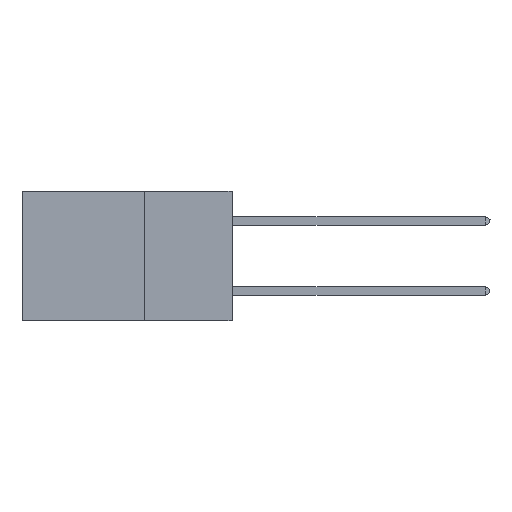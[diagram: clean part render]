
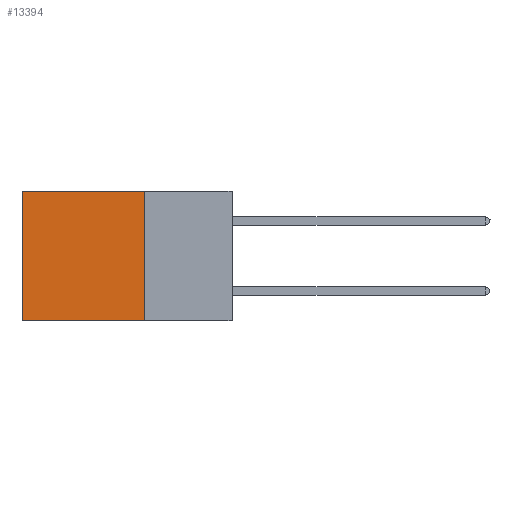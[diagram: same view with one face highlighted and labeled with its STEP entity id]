
A CAD part, left-side view. The second image highlights one B-rep face of the part: STEP entity #13394.
In plain terms, the highlighted planar face has unit normal (-1, 0, 0).
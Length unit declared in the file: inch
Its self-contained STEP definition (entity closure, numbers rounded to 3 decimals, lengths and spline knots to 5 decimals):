
#149 = CARTESIAN_POINT ( 'NONE',  ( 0.2875, 0.25, -0.37 ) ) ;
#176 = VERTEX_POINT ( 'NONE', #1480 ) ;
#900 = ORIENTED_EDGE ( 'NONE', *, *, #16935, .T. ) ;
#1480 = CARTESIAN_POINT ( 'NONE',  ( 0.2875, 0.6, -0.37 ) ) ;
#4264 = EDGE_CURVE ( 'NONE', #11045, #176, #23372, .T. ) ;
#4850 = EDGE_CURVE ( 'NONE', #27379, #11045, #20288, .T. ) ;
#5281 = CARTESIAN_POINT ( 'NONE',  ( 0.2875, 0.6, 0. ) ) ;
#5306 = VERTEX_POINT ( 'NONE', #5281 ) ;
#5441 = VECTOR ( 'NONE', #6538, 39.37008 ) ;
#5892 = ORIENTED_EDGE ( 'NONE', *, *, #22264, .T. ) ;
#6002 = CARTESIAN_POINT ( 'NONE',  ( 0.2875, 0.25, -0.37 ) ) ;
#6138 = LINE ( 'NONE', #17353, #5441 ) ;
#6538 = DIRECTION ( 'NONE',  ( 0., 0., -1. ) ) ;
#7806 = DIRECTION ( 'NONE',  ( 0., 0., -1. ) ) ;
#10648 = VECTOR ( 'NONE', #22127, 39.37008 ) ;
#11045 = VERTEX_POINT ( 'NONE', #149 ) ;
#11805 = CARTESIAN_POINT ( 'NONE',  ( 0.2875, 0.25, 0. ) ) ;
#11829 = VECTOR ( 'NONE', #21211, 39.37008 ) ;
#11970 = ORIENTED_EDGE ( 'NONE', *, *, #4264, .F. ) ;
#12078 = CARTESIAN_POINT ( 'NONE',  ( 0.2875, 0.25, 0. ) ) ;
#13394 = ADVANCED_FACE ( 'NONE', ( #25470 ), #18605, .F. ) ;
#14545 = VECTOR ( 'NONE', #19078, 39.37008 ) ;
#14740 = CARTESIAN_POINT ( 'NONE',  ( 0.2875, 0.25, 0. ) ) ;
#16935 = EDGE_CURVE ( 'NONE', #5306, #176, #6138, .T. ) ;
#17353 = CARTESIAN_POINT ( 'NONE',  ( 0.2875, 0.6, 0. ) ) ;
#18605 = PLANE ( 'NONE',  #22738 ) ;
#19078 = DIRECTION ( 'NONE',  ( 0., 0., -1. ) ) ;
#20288 = LINE ( 'NONE', #14740, #14545 ) ;
#20792 = DIRECTION ( 'NONE',  ( 1., 0., 0. ) ) ;
#21211 = DIRECTION ( 'NONE',  ( 0., 1., 0. ) ) ;
#22127 = DIRECTION ( 'NONE',  ( 0., 1., 0. ) ) ;
#22264 = EDGE_CURVE ( 'NONE', #27379, #5306, #27968, .T. ) ;
#22738 = AXIS2_PLACEMENT_3D ( 'NONE', #12078, #20792, #7806 ) ;
#23372 = LINE ( 'NONE', #6002, #11829 ) ;
#24262 = CARTESIAN_POINT ( 'NONE',  ( 0.2875, 0.25, 0. ) ) ;
#25470 = FACE_OUTER_BOUND ( 'NONE', #27580, .T. ) ;
#27379 = VERTEX_POINT ( 'NONE', #11805 ) ;
#27580 = EDGE_LOOP ( 'NONE', ( #900, #11970, #28067, #5892 ) ) ;
#27968 = LINE ( 'NONE', #24262, #10648 ) ;
#28067 = ORIENTED_EDGE ( 'NONE', *, *, #4850, .F. ) ;
